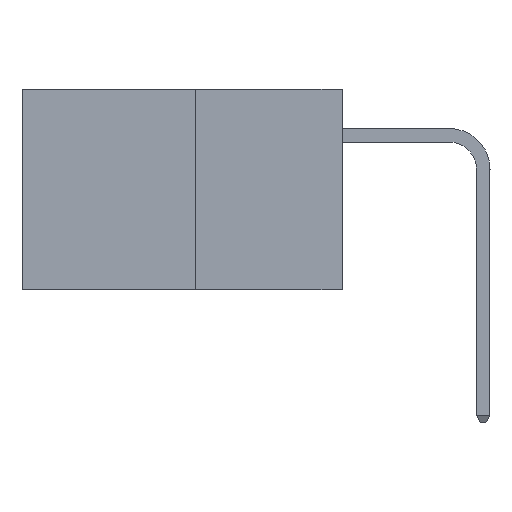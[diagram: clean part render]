
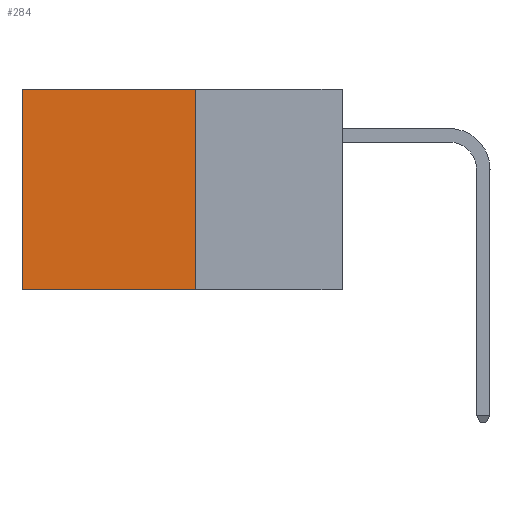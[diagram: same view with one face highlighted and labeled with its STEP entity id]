
A CAD part, left-side view. The second image highlights one B-rep face of the part: STEP entity #284.
In plain terms, the highlighted planar face has unit normal (-1, 0, 0).
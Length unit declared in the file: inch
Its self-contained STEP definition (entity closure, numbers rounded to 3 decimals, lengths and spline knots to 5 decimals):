
#272 = VERTEX_POINT ( 'NONE', #6655 ) ;
#284 = ADVANCED_FACE ( 'NONE', ( #3047 ), #15078, .F. ) ;
#601 = DIRECTION ( 'NONE',  ( 1., 0., 0. ) ) ;
#746 = CARTESIAN_POINT ( 'NONE',  ( 0.277, 0.27, -0.37 ) ) ;
#779 = CARTESIAN_POINT ( 'NONE',  ( 0.277, 0.27, -0.37 ) ) ;
#1434 = DIRECTION ( 'NONE',  ( 0., 0., -1. ) ) ;
#2239 = EDGE_CURVE ( 'NONE', #272, #11830, #3433, .T. ) ;
#2653 = CARTESIAN_POINT ( 'NONE',  ( 0.277, 0.59, -0.37 ) ) ;
#2819 = DIRECTION ( 'NONE',  ( 0., 1., 0. ) ) ;
#3047 = FACE_OUTER_BOUND ( 'NONE', #13899, .T. ) ;
#3069 = CARTESIAN_POINT ( 'NONE',  ( 0.277, 0.27, 0. ) ) ;
#3433 = LINE ( 'NONE', #779, #17870 ) ;
#3562 = EDGE_CURVE ( 'NONE', #14693, #11830, #9358, .T. ) ;
#4290 = CARTESIAN_POINT ( 'NONE',  ( 0.277, 0.27, 0. ) ) ;
#4480 = AXIS2_PLACEMENT_3D ( 'NONE', #6297, #601, #1434 ) ;
#6297 = CARTESIAN_POINT ( 'NONE',  ( 0.277, 0.27, -0.37 ) ) ;
#6655 = CARTESIAN_POINT ( 'NONE',  ( 0.277, 0.27, -0.37 ) ) ;
#6775 = DIRECTION ( 'NONE',  ( 0., 0., -1. ) ) ;
#7078 = VECTOR ( 'NONE', #12865, 39.37008 ) ;
#7585 = LINE ( 'NONE', #746, #14599 ) ;
#9088 = CARTESIAN_POINT ( 'NONE',  ( 0.277, 0.59, -0.37 ) ) ;
#9356 = VERTEX_POINT ( 'NONE', #4290 ) ;
#9358 = LINE ( 'NONE', #2653, #13512 ) ;
#11177 = CARTESIAN_POINT ( 'NONE',  ( 0.277, 0.59, 0. ) ) ;
#11830 = VERTEX_POINT ( 'NONE', #9088 ) ;
#12073 = DIRECTION ( 'NONE',  ( 0., 0., -1. ) ) ;
#12354 = EDGE_CURVE ( 'NONE', #9356, #14693, #12918, .T. ) ;
#12865 = DIRECTION ( 'NONE',  ( 0., 1., 0. ) ) ;
#12918 = LINE ( 'NONE', #3069, #7078 ) ;
#13512 = VECTOR ( 'NONE', #6775, 39.37008 ) ;
#13899 = EDGE_LOOP ( 'NONE', ( #15451, #15218, #15010, #14990 ) ) ;
#14599 = VECTOR ( 'NONE', #12073, 39.37008 ) ;
#14693 = VERTEX_POINT ( 'NONE', #11177 ) ;
#14990 = ORIENTED_EDGE ( 'NONE', *, *, #12354, .T. ) ;
#15010 = ORIENTED_EDGE ( 'NONE', *, *, #16982, .F. ) ;
#15078 = PLANE ( 'NONE',  #4480 ) ;
#15218 = ORIENTED_EDGE ( 'NONE', *, *, #2239, .F. ) ;
#15451 = ORIENTED_EDGE ( 'NONE', *, *, #3562, .T. ) ;
#16982 = EDGE_CURVE ( 'NONE', #9356, #272, #7585, .T. ) ;
#17870 = VECTOR ( 'NONE', #2819, 39.37008 ) ;
